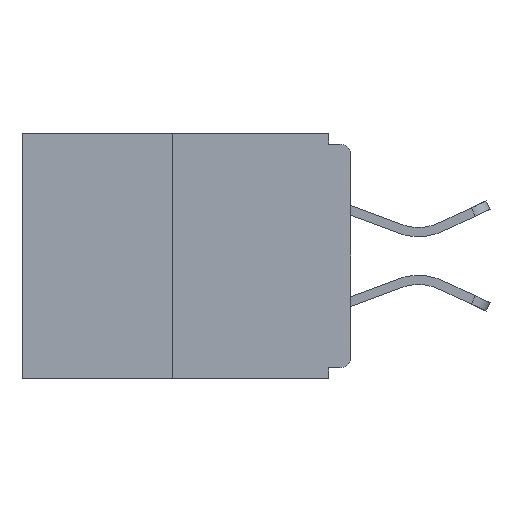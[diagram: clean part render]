
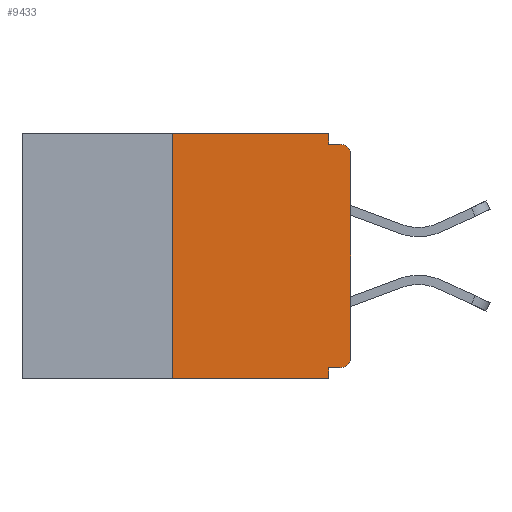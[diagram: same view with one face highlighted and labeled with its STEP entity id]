
A CAD part, left-side view. The second image highlights one B-rep face of the part: STEP entity #9433.
In plain terms, the highlighted planar face has unit normal (-1, 0, 0).
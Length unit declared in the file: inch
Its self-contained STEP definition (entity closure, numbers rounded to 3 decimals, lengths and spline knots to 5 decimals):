
#291 = DIRECTION ( 'NONE',  ( -1., 0., 0. ) ) ;
#432 = ORIENTED_EDGE ( 'NONE', *, *, #13325, .T. ) ;
#550 = EDGE_LOOP ( 'NONE', ( #5397, #4375, #8811, #13626, #12825, #4054, #432, #12681, #12254, #14329 ) ) ;
#953 = CARTESIAN_POINT ( 'NONE',  ( 0., 0., -0.03 ) ) ;
#1042 = EDGE_CURVE ( 'NONE', #16790, #8643, #2424, .T. ) ;
#1223 = CARTESIAN_POINT ( 'NONE',  ( 0., 0.031, -0.343 ) ) ;
#1505 = VECTOR ( 'NONE', #13119, 39.37008 ) ;
#1726 = DIRECTION ( 'NONE',  ( 0., -1., 0. ) ) ;
#2012 = CARTESIAN_POINT ( 'NONE',  ( 0., 0.015, -0.015 ) ) ;
#2068 = VERTEX_POINT ( 'NONE', #2012 ) ;
#2424 = LINE ( 'NONE', #6946, #16493 ) ;
#2674 = EDGE_CURVE ( 'NONE', #16270, #12293, #14959, .T. ) ;
#2722 = CARTESIAN_POINT ( 'NONE',  ( 0., 0.015, -0.328 ) ) ;
#2855 = DIRECTION ( 'NONE',  ( -1., 0., 0. ) ) ;
#2987 = LINE ( 'NONE', #16265, #9008 ) ;
#3180 = VECTOR ( 'NONE', #3949, 39.37008 ) ;
#3415 = DIRECTION ( 'NONE',  ( 0., 0., -1. ) ) ;
#3709 = EDGE_CURVE ( 'NONE', #6928, #7599, #10811, .T. ) ;
#3949 = DIRECTION ( 'NONE',  ( 0., 0., 1. ) ) ;
#4054 = ORIENTED_EDGE ( 'NONE', *, *, #2674, .T. ) ;
#4375 = ORIENTED_EDGE ( 'NONE', *, *, #13702, .F. ) ;
#4382 = VERTEX_POINT ( 'NONE', #15964 ) ;
#5397 = ORIENTED_EDGE ( 'NONE', *, *, #1042, .F. ) ;
#5462 = VECTOR ( 'NONE', #3415, 39.37008 ) ;
#5841 = AXIS2_PLACEMENT_3D ( 'NONE', #15173, #7279, #12600 ) ;
#5881 = EDGE_CURVE ( 'NONE', #4382, #7599, #11176, .T. ) ;
#6047 = CARTESIAN_POINT ( 'NONE',  ( 0., 0.46, -0.343 ) ) ;
#6144 = LINE ( 'NONE', #9248, #7996 ) ;
#6184 = EDGE_CURVE ( 'NONE', #16270, #6928, #10745, .T. ) ;
#6920 = DIRECTION ( 'NONE',  ( 0., 0., 1. ) ) ;
#6928 = VERTEX_POINT ( 'NONE', #15856 ) ;
#6946 = CARTESIAN_POINT ( 'NONE',  ( 0., 0.46, 0. ) ) ;
#7216 = VECTOR ( 'NONE', #15918, 39.37008 ) ;
#7279 = DIRECTION ( 'NONE',  ( 1., 0., 0. ) ) ;
#7447 = PLANE ( 'NONE',  #5841 ) ;
#7599 = VERTEX_POINT ( 'NONE', #16183 ) ;
#7996 = VECTOR ( 'NONE', #12011, 39.37008 ) ;
#8379 = LINE ( 'NONE', #11957, #3180 ) ;
#8643 = VERTEX_POINT ( 'NONE', #11627 ) ;
#8764 = DIRECTION ( 'NONE',  ( 0., -1., 0. ) ) ;
#8811 = ORIENTED_EDGE ( 'NONE', *, *, #5881, .T. ) ;
#8815 = CIRCLE ( 'NONE', #9427, 0.015 ) ;
#9008 = VECTOR ( 'NONE', #6920, 39.37008 ) ;
#9214 = VERTEX_POINT ( 'NONE', #953 ) ;
#9248 = CARTESIAN_POINT ( 'NONE',  ( 0., 0., -0.015 ) ) ;
#9284 = CARTESIAN_POINT ( 'NONE',  ( 0., 0., -0.328 ) ) ;
#9427 = AXIS2_PLACEMENT_3D ( 'NONE', #12002, #2855, #13539 ) ;
#9433 = ADVANCED_FACE ( 'NONE', ( #10956 ), #7447, .F. ) ;
#9929 = VECTOR ( 'NONE', #8764, 39.37008 ) ;
#10209 = LINE ( 'NONE', #16721, #5462 ) ;
#10329 = CARTESIAN_POINT ( 'NONE',  ( 0., 0., -0.313 ) ) ;
#10522 = EDGE_CURVE ( 'NONE', #14702, #2068, #6144, .T. ) ;
#10745 = LINE ( 'NONE', #9284, #7216 ) ;
#10811 = LINE ( 'NONE', #1223, #1505 ) ;
#10900 = EDGE_CURVE ( 'NONE', #9214, #2068, #8815, .T. ) ;
#10956 = FACE_OUTER_BOUND ( 'NONE', #550, .T. ) ;
#11176 = LINE ( 'NONE', #6047, #9929 ) ;
#11627 = CARTESIAN_POINT ( 'NONE',  ( 0., 0.031, 0. ) ) ;
#11957 = CARTESIAN_POINT ( 'NONE',  ( 0., 0.25, 0. ) ) ;
#11958 = DIRECTION ( 'NONE',  ( 0., 0., -1. ) ) ;
#12002 = CARTESIAN_POINT ( 'NONE',  ( 0., 0.015, -0.03 ) ) ;
#12011 = DIRECTION ( 'NONE',  ( 0., -1., 0. ) ) ;
#12254 = ORIENTED_EDGE ( 'NONE', *, *, #10522, .F. ) ;
#12293 = VERTEX_POINT ( 'NONE', #10329 ) ;
#12600 = DIRECTION ( 'NONE',  ( 0., 0., -1. ) ) ;
#12681 = ORIENTED_EDGE ( 'NONE', *, *, #10900, .T. ) ;
#12825 = ORIENTED_EDGE ( 'NONE', *, *, #6184, .F. ) ;
#13119 = DIRECTION ( 'NONE',  ( 0., 0., -1. ) ) ;
#13325 = EDGE_CURVE ( 'NONE', #12293, #9214, #2987, .T. ) ;
#13539 = DIRECTION ( 'NONE',  ( 0., 0., -1. ) ) ;
#13626 = ORIENTED_EDGE ( 'NONE', *, *, #3709, .F. ) ;
#13702 = EDGE_CURVE ( 'NONE', #4382, #16790, #8379, .T. ) ;
#14072 = EDGE_CURVE ( 'NONE', #8643, #14702, #10209, .T. ) ;
#14219 = CARTESIAN_POINT ( 'NONE',  ( 0., 0.25, 0. ) ) ;
#14329 = ORIENTED_EDGE ( 'NONE', *, *, #14072, .F. ) ;
#14702 = VERTEX_POINT ( 'NONE', #15707 ) ;
#14959 = CIRCLE ( 'NONE', #16301, 0.015 ) ;
#15173 = CARTESIAN_POINT ( 'NONE',  ( 0., 0.46, 0. ) ) ;
#15707 = CARTESIAN_POINT ( 'NONE',  ( 0., 0.031, -0.015 ) ) ;
#15856 = CARTESIAN_POINT ( 'NONE',  ( 0., 0.031, -0.328 ) ) ;
#15918 = DIRECTION ( 'NONE',  ( 0., 1., 0. ) ) ;
#15964 = CARTESIAN_POINT ( 'NONE',  ( 0., 0.25, -0.343 ) ) ;
#16168 = CARTESIAN_POINT ( 'NONE',  ( 0., 0.015, -0.313 ) ) ;
#16183 = CARTESIAN_POINT ( 'NONE',  ( 0., 0.031, -0.343 ) ) ;
#16265 = CARTESIAN_POINT ( 'NONE',  ( 0., 0., 0. ) ) ;
#16270 = VERTEX_POINT ( 'NONE', #2722 ) ;
#16301 = AXIS2_PLACEMENT_3D ( 'NONE', #16168, #291, #11958 ) ;
#16493 = VECTOR ( 'NONE', #1726, 39.37008 ) ;
#16721 = CARTESIAN_POINT ( 'NONE',  ( 0., 0.031, 0. ) ) ;
#16790 = VERTEX_POINT ( 'NONE', #14219 ) ;
